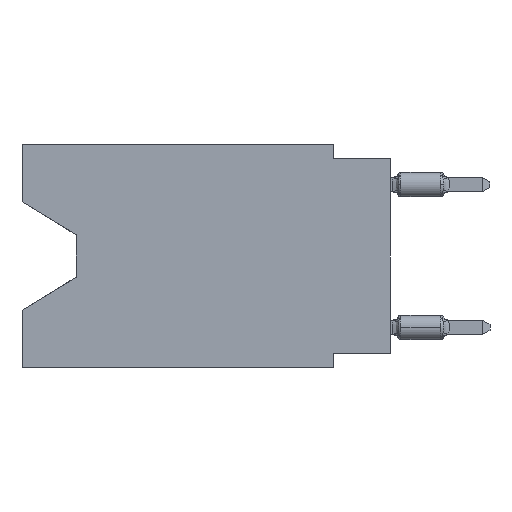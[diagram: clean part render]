
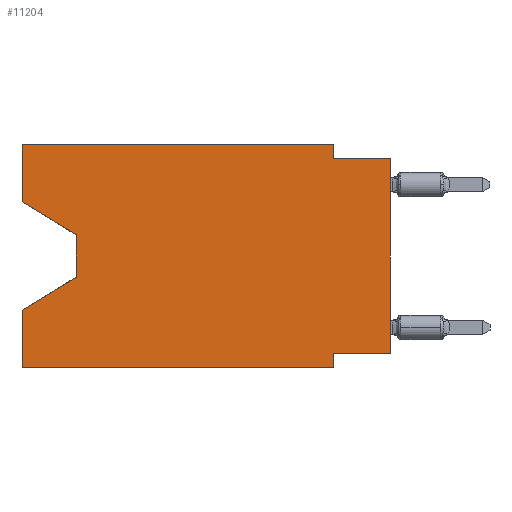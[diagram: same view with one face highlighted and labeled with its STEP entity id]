
A CAD part, left-side view. The second image highlights one B-rep face of the part: STEP entity #11204.
In plain terms, the highlighted planar face has unit normal (-1, 0, 0).
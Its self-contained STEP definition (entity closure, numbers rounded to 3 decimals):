
#6 = CARTESIAN_POINT ( 'NONE',  ( 0., 2.54, 0. ) ) ;
#175 = ORIENTED_EDGE ( 'NONE', *, *, #1301, .F. ) ;
#291 = VERTEX_POINT ( 'NONE', #17858 ) ;
#881 = CARTESIAN_POINT ( 'NONE',  ( 0., 2.54, -9.271 ) ) ;
#1193 = VECTOR ( 'NONE', #19226, 1000. ) ;
#1220 = EDGE_CURVE ( 'NONE', #5441, #13567, #6788, .T. ) ;
#1301 = EDGE_CURVE ( 'NONE', #5551, #14432, #10411, .T. ) ;
#1407 = DIRECTION ( 'NONE',  ( 1., 0., 0. ) ) ;
#1410 = CARTESIAN_POINT ( 'NONE',  ( 0., 16.383, 0. ) ) ;
#1581 = ORIENTED_EDGE ( 'NONE', *, *, #1220, .F. ) ;
#1707 = EDGE_CURVE ( 'NONE', #14432, #12492, #12198, .T. ) ;
#1730 = CARTESIAN_POINT ( 'NONE',  ( 0., 13.97, -5.893 ) ) ;
#1989 = LINE ( 'NONE', #9466, #14977 ) ;
#2198 = EDGE_CURVE ( 'NONE', #9615, #291, #8309, .T. ) ;
#2236 = VECTOR ( 'NONE', #6167, 1000. ) ;
#2258 = LINE ( 'NONE', #17421, #6359 ) ;
#2828 = LINE ( 'NONE', #1410, #2236 ) ;
#3089 = CARTESIAN_POINT ( 'NONE',  ( 0., 13.97, -4.013 ) ) ;
#3513 = DIRECTION ( 'NONE',  ( 0., 0., 1. ) ) ;
#3553 = CARTESIAN_POINT ( 'NONE',  ( 0., 13.97, -5.893 ) ) ;
#3855 = ORIENTED_EDGE ( 'NONE', *, *, #6396, .T. ) ;
#4046 = CARTESIAN_POINT ( 'NONE',  ( 0., 16.383, -2.546 ) ) ;
#4209 = DIRECTION ( 'NONE',  ( 0., 1., 0. ) ) ;
#5039 = LINE ( 'NONE', #13832, #6858 ) ;
#5158 = ORIENTED_EDGE ( 'NONE', *, *, #14228, .T. ) ;
#5256 = CARTESIAN_POINT ( 'NONE',  ( 0., 16.383, -9.906 ) ) ;
#5302 = CARTESIAN_POINT ( 'NONE',  ( 0., 2.54, -9.906 ) ) ;
#5374 = ORIENTED_EDGE ( 'NONE', *, *, #11363, .T. ) ;
#5441 = VERTEX_POINT ( 'NONE', #881 ) ;
#5466 = ORIENTED_EDGE ( 'NONE', *, *, #7988, .F. ) ;
#5551 = VERTEX_POINT ( 'NONE', #7231 ) ;
#5702 = VERTEX_POINT ( 'NONE', #3089 ) ;
#6167 = DIRECTION ( 'NONE',  ( 0., -1., 0. ) ) ;
#6359 = VECTOR ( 'NONE', #17330, 1000. ) ;
#6396 = EDGE_CURVE ( 'NONE', #11086, #5702, #7185, .T. ) ;
#6571 = CARTESIAN_POINT ( 'NONE',  ( 0., 0., -0.635 ) ) ;
#6620 = ORIENTED_EDGE ( 'NONE', *, *, #2198, .T. ) ;
#6745 = VERTEX_POINT ( 'NONE', #15837 ) ;
#6788 = LINE ( 'NONE', #13038, #1193 ) ;
#6794 = CARTESIAN_POINT ( 'NONE',  ( 0., 16.383, 0. ) ) ;
#6858 = VECTOR ( 'NONE', #12309, 1000. ) ;
#7037 = VECTOR ( 'NONE', #8598, 1000. ) ;
#7082 = DIRECTION ( 'NONE',  ( 0., 0., 1. ) ) ;
#7185 = LINE ( 'NONE', #10415, #7037 ) ;
#7231 = CARTESIAN_POINT ( 'NONE',  ( 0., 2.54, 0. ) ) ;
#7366 = CARTESIAN_POINT ( 'NONE',  ( 0., 0., -9.271 ) ) ;
#7652 = CARTESIAN_POINT ( 'NONE',  ( 0., 2.54, -0.635 ) ) ;
#7988 = EDGE_CURVE ( 'NONE', #6745, #5551, #2828, .T. ) ;
#8096 = DIRECTION ( 'NONE',  ( 0., 0.855, -0.519 ) ) ;
#8309 = LINE ( 'NONE', #3553, #8867 ) ;
#8434 = EDGE_CURVE ( 'NONE', #5702, #9615, #2258, .T. ) ;
#8598 = DIRECTION ( 'NONE',  ( 0., -0.855, -0.519 ) ) ;
#8867 = VECTOR ( 'NONE', #8096, 1000. ) ;
#9089 = VECTOR ( 'NONE', #4209, 1000. ) ;
#9466 = CARTESIAN_POINT ( 'NONE',  ( 0., 16.383, 0. ) ) ;
#9615 = VERTEX_POINT ( 'NONE', #1730 ) ;
#10411 = LINE ( 'NONE', #6, #18325 ) ;
#10415 = CARTESIAN_POINT ( 'NONE',  ( 0., 16.383, -2.546 ) ) ;
#10886 = ORIENTED_EDGE ( 'NONE', *, *, #8434, .T. ) ;
#10983 = DIRECTION ( 'NONE',  ( 0., 0., 1. ) ) ;
#10990 = LINE ( 'NONE', #18592, #19095 ) ;
#11086 = VERTEX_POINT ( 'NONE', #4046 ) ;
#11204 = ADVANCED_FACE ( 'NONE', ( #16478 ), #18397, .F. ) ;
#11363 = EDGE_CURVE ( 'NONE', #12543, #13567, #5039, .T. ) ;
#11482 = ORIENTED_EDGE ( 'NONE', *, *, #18978, .F. ) ;
#11894 = LINE ( 'NONE', #13799, #9089 ) ;
#11921 = DIRECTION ( 'NONE',  ( 0., 0., -1. ) ) ;
#12198 = LINE ( 'NONE', #15244, #14011 ) ;
#12309 = DIRECTION ( 'NONE',  ( 0., -1., 0. ) ) ;
#12492 = VERTEX_POINT ( 'NONE', #6571 ) ;
#12543 = VERTEX_POINT ( 'NONE', #5256 ) ;
#13038 = CARTESIAN_POINT ( 'NONE',  ( 0., 2.54, -9.906 ) ) ;
#13236 = LINE ( 'NONE', #6794, #17259 ) ;
#13480 = ORIENTED_EDGE ( 'NONE', *, *, #1707, .F. ) ;
#13567 = VERTEX_POINT ( 'NONE', #5302 ) ;
#13718 = DIRECTION ( 'NONE',  ( 0., -1., 0. ) ) ;
#13799 = CARTESIAN_POINT ( 'NONE',  ( 0., 0., -9.271 ) ) ;
#13832 = CARTESIAN_POINT ( 'NONE',  ( 0., 16.383, -9.906 ) ) ;
#14011 = VECTOR ( 'NONE', #13718, 1000. ) ;
#14228 = EDGE_CURVE ( 'NONE', #16667, #12492, #10990, .T. ) ;
#14432 = VERTEX_POINT ( 'NONE', #7652 ) ;
#14452 = EDGE_CURVE ( 'NONE', #16667, #5441, #11894, .T. ) ;
#14977 = VECTOR ( 'NONE', #10983, 1000. ) ;
#15244 = CARTESIAN_POINT ( 'NONE',  ( 0., 0., -0.635 ) ) ;
#15254 = EDGE_LOOP ( 'NONE', ( #3855, #10886, #6620, #11482, #5374, #1581, #15550, #5158, #13480, #175, #5466, #19937 ) ) ;
#15550 = ORIENTED_EDGE ( 'NONE', *, *, #14452, .F. ) ;
#15837 = CARTESIAN_POINT ( 'NONE',  ( 0., 16.383, 0. ) ) ;
#16478 = FACE_OUTER_BOUND ( 'NONE', #15254, .T. ) ;
#16667 = VERTEX_POINT ( 'NONE', #7366 ) ;
#16781 = DIRECTION ( 'NONE',  ( 0., 0., -1. ) ) ;
#16813 = EDGE_CURVE ( 'NONE', #11086, #6745, #1989, .T. ) ;
#17259 = VECTOR ( 'NONE', #7082, 1000. ) ;
#17330 = DIRECTION ( 'NONE',  ( 0., 0., -1. ) ) ;
#17421 = CARTESIAN_POINT ( 'NONE',  ( 0., 13.97, -4.013 ) ) ;
#17832 = AXIS2_PLACEMENT_3D ( 'NONE', #18196, #1407, #11921 ) ;
#17858 = CARTESIAN_POINT ( 'NONE',  ( 0., 16.383, -7.36 ) ) ;
#18196 = CARTESIAN_POINT ( 'NONE',  ( 0., 16.383, 0. ) ) ;
#18325 = VECTOR ( 'NONE', #16781, 1000. ) ;
#18397 = PLANE ( 'NONE',  #17832 ) ;
#18592 = CARTESIAN_POINT ( 'NONE',  ( 0., 0., 0. ) ) ;
#18978 = EDGE_CURVE ( 'NONE', #12543, #291, #13236, .T. ) ;
#19095 = VECTOR ( 'NONE', #3513, 1000. ) ;
#19226 = DIRECTION ( 'NONE',  ( 0., 0., -1. ) ) ;
#19937 = ORIENTED_EDGE ( 'NONE', *, *, #16813, .F. ) ;
